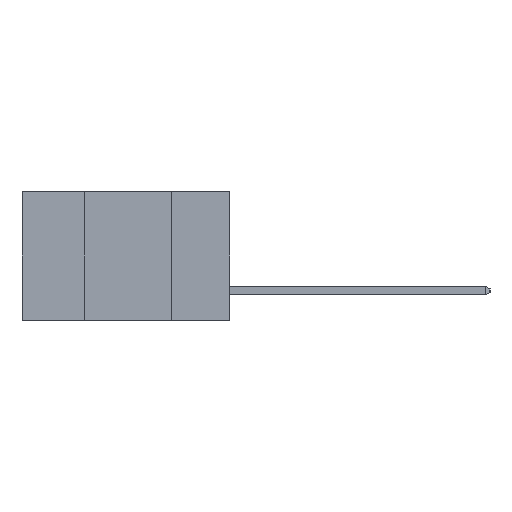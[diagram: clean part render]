
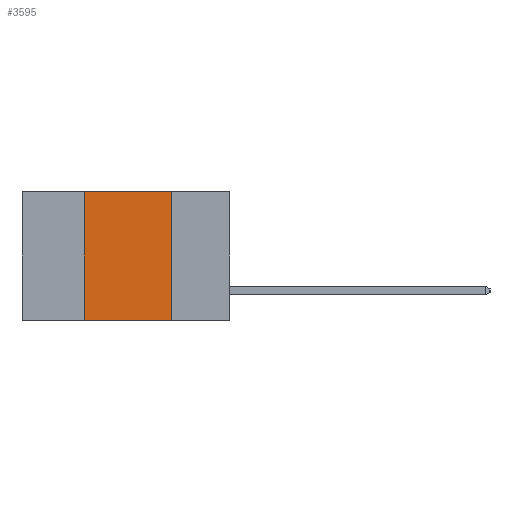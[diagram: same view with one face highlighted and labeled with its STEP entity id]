
A CAD part, left-side view. The second image highlights one B-rep face of the part: STEP entity #3595.
In plain terms, the highlighted planar face has unit normal (-1, 0, 0).
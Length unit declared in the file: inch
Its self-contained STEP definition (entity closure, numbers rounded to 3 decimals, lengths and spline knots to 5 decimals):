
#563 = CARTESIAN_POINT ( 'NONE',  ( 0., 0.6, -0.37 ) ) ;
#759 = EDGE_CURVE ( 'NONE', #3571, #4351, #8174, .T. ) ;
#1177 = EDGE_LOOP ( 'NONE', ( #6997, #3454, #4389, #2454 ) ) ;
#1457 = DIRECTION ( 'NONE',  ( 0., -1., 0. ) ) ;
#1772 = VECTOR ( 'NONE', #10459, 39.37008 ) ;
#2454 = ORIENTED_EDGE ( 'NONE', *, *, #759, .T. ) ;
#3454 = ORIENTED_EDGE ( 'NONE', *, *, #6649, .F. ) ;
#3571 = VERTEX_POINT ( 'NONE', #12311 ) ;
#3595 = ADVANCED_FACE ( 'NONE', ( #15047 ), #6290, .F. ) ;
#4311 = CARTESIAN_POINT ( 'NONE',  ( 0., 0.17, -0.37 ) ) ;
#4351 = VERTEX_POINT ( 'NONE', #8852 ) ;
#4377 = LINE ( 'NONE', #7201, #4777 ) ;
#4389 = ORIENTED_EDGE ( 'NONE', *, *, #5013, .F. ) ;
#4462 = VERTEX_POINT ( 'NONE', #12684 ) ;
#4720 = LINE ( 'NONE', #15163, #1772 ) ;
#4777 = VECTOR ( 'NONE', #14440, 39.37008 ) ;
#5013 = EDGE_CURVE ( 'NONE', #3571, #9543, #4377, .T. ) ;
#5555 = DIRECTION ( 'NONE',  ( 0., 0., -1. ) ) ;
#6290 = PLANE ( 'NONE',  #15001 ) ;
#6649 = EDGE_CURVE ( 'NONE', #9543, #4462, #4720, .T. ) ;
#6997 = ORIENTED_EDGE ( 'NONE', *, *, #15574, .F. ) ;
#7201 = CARTESIAN_POINT ( 'NONE',  ( 0., 0.42, -0.37 ) ) ;
#7521 = CARTESIAN_POINT ( 'NONE',  ( 0., 0.6, 0. ) ) ;
#8174 = LINE ( 'NONE', #563, #14204 ) ;
#8766 = DIRECTION ( 'NONE',  ( 0., 0., -1. ) ) ;
#8852 = CARTESIAN_POINT ( 'NONE',  ( 0., 0.17, -0.37 ) ) ;
#9201 = VECTOR ( 'NONE', #5555, 39.37008 ) ;
#9543 = VERTEX_POINT ( 'NONE', #14216 ) ;
#10459 = DIRECTION ( 'NONE',  ( 0., -1., 0. ) ) ;
#12311 = CARTESIAN_POINT ( 'NONE',  ( 0., 0.42, -0.37 ) ) ;
#12684 = CARTESIAN_POINT ( 'NONE',  ( 0., 0.17, 0. ) ) ;
#14204 = VECTOR ( 'NONE', #1457, 39.37008 ) ;
#14216 = CARTESIAN_POINT ( 'NONE',  ( 0., 0.42, 0. ) ) ;
#14440 = DIRECTION ( 'NONE',  ( 0., 0., 1. ) ) ;
#15001 = AXIS2_PLACEMENT_3D ( 'NONE', #7521, #15128, #8766 ) ;
#15047 = FACE_OUTER_BOUND ( 'NONE', #1177, .T. ) ;
#15128 = DIRECTION ( 'NONE',  ( 1., 0., 0. ) ) ;
#15163 = CARTESIAN_POINT ( 'NONE',  ( 0., 0.6, 0. ) ) ;
#15574 = EDGE_CURVE ( 'NONE', #4462, #4351, #15604, .T. ) ;
#15604 = LINE ( 'NONE', #4311, #9201 ) ;
